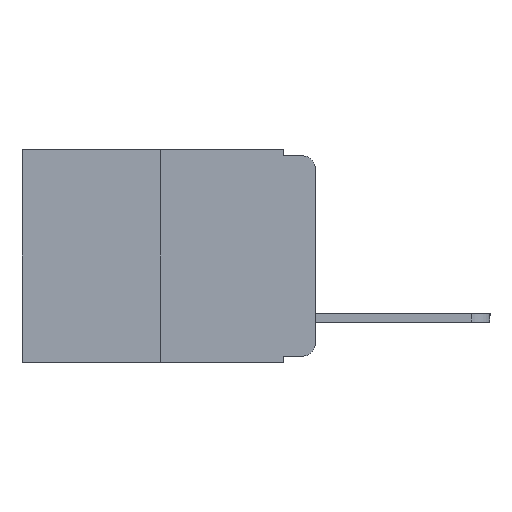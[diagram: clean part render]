
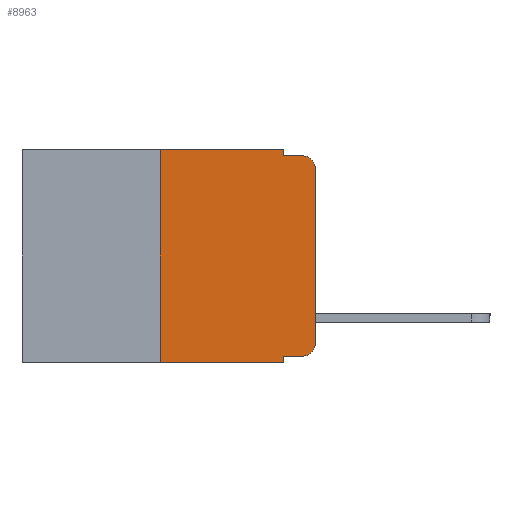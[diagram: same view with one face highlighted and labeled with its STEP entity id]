
A CAD part, left-side view. The second image highlights one B-rep face of the part: STEP entity #8963.
In plain terms, the highlighted planar face has unit normal (-1, 0, 0).
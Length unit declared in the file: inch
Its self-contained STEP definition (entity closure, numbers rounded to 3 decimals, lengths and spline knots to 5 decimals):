
#248 = CARTESIAN_POINT ( 'NONE',  ( 0., 0.02, -0.01 ) ) ;
#283 = VECTOR ( 'NONE', #9025, 39.37008 ) ;
#337 = CARTESIAN_POINT ( 'NONE',  ( 0., 0., -0.03 ) ) ;
#573 = LINE ( 'NONE', #3915, #283 ) ;
#720 = CARTESIAN_POINT ( 'NONE',  ( 0., 0.051, -0.01 ) ) ;
#937 = VECTOR ( 'NONE', #6327, 39.37008 ) ;
#947 = DIRECTION ( 'NONE',  ( 0., -1., 0. ) ) ;
#1385 = ORIENTED_EDGE ( 'NONE', *, *, #1768, .F. ) ;
#1392 = CARTESIAN_POINT ( 'NONE',  ( 0., 0.02, -0.03 ) ) ;
#1399 = VERTEX_POINT ( 'NONE', #7444 ) ;
#1763 = CARTESIAN_POINT ( 'NONE',  ( 0., 0., -0.313 ) ) ;
#1768 = EDGE_CURVE ( 'NONE', #5546, #5086, #3688, .T. ) ;
#1831 = CARTESIAN_POINT ( 'NONE',  ( 0., 0.051, -0.333 ) ) ;
#2217 = LINE ( 'NONE', #4560, #6785 ) ;
#2293 = VECTOR ( 'NONE', #9776, 39.37008 ) ;
#2401 = VERTEX_POINT ( 'NONE', #8206 ) ;
#2758 = EDGE_CURVE ( 'NONE', #6033, #5086, #10913, .T. ) ;
#2836 = CARTESIAN_POINT ( 'NONE',  ( 0., 0.25, 0. ) ) ;
#2842 = CARTESIAN_POINT ( 'NONE',  ( 0., 0.051, 0. ) ) ;
#2931 = VERTEX_POINT ( 'NONE', #1831 ) ;
#3153 = CARTESIAN_POINT ( 'NONE',  ( 0., 0.051, -0.343 ) ) ;
#3379 = EDGE_CURVE ( 'NONE', #5992, #6033, #8115, .T. ) ;
#3432 = PLANE ( 'NONE',  #9098 ) ;
#3538 = EDGE_CURVE ( 'NONE', #1399, #5992, #3868, .T. ) ;
#3688 = LINE ( 'NONE', #9476, #937 ) ;
#3834 = CARTESIAN_POINT ( 'NONE',  ( 0., 0.051, 0. ) ) ;
#3868 = CIRCLE ( 'NONE', #10484, 0.02 ) ;
#3899 = VERTEX_POINT ( 'NONE', #3153 ) ;
#3915 = CARTESIAN_POINT ( 'NONE',  ( 0., 0.051, -0.333 ) ) ;
#3979 = DIRECTION ( 'NONE',  ( 0., 0., -1. ) ) ;
#4302 = CARTESIAN_POINT ( 'NONE',  ( 0., 0.25, -0.343 ) ) ;
#4360 = EDGE_CURVE ( 'NONE', #2931, #1399, #573, .T. ) ;
#4463 = DIRECTION ( 'NONE',  ( 0., 0., 1. ) ) ;
#4489 = CARTESIAN_POINT ( 'NONE',  ( 0., 0., 0. ) ) ;
#4560 = CARTESIAN_POINT ( 'NONE',  ( 0., 0.25, 0. ) ) ;
#4561 = ORIENTED_EDGE ( 'NONE', *, *, #10525, .T. ) ;
#5086 = VERTEX_POINT ( 'NONE', #248 ) ;
#5288 = DIRECTION ( 'NONE',  ( 0., 0., -1. ) ) ;
#5478 = EDGE_CURVE ( 'NONE', #10217, #10529, #2217, .T. ) ;
#5546 = VERTEX_POINT ( 'NONE', #720 ) ;
#5595 = CARTESIAN_POINT ( 'NONE',  ( 0., 0.473, -0.343 ) ) ;
#5602 = EDGE_CURVE ( 'NONE', #2931, #3899, #10116, .T. ) ;
#5877 = VECTOR ( 'NONE', #947, 39.37008 ) ;
#5992 = VERTEX_POINT ( 'NONE', #1763 ) ;
#6033 = VERTEX_POINT ( 'NONE', #337 ) ;
#6080 = ORIENTED_EDGE ( 'NONE', *, *, #3379, .T. ) ;
#6327 = DIRECTION ( 'NONE',  ( 0., -1., 0. ) ) ;
#6343 = ORIENTED_EDGE ( 'NONE', *, *, #8007, .F. ) ;
#6396 = VECTOR ( 'NONE', #10530, 39.37008 ) ;
#6617 = ORIENTED_EDGE ( 'NONE', *, *, #10565, .F. ) ;
#6785 = VECTOR ( 'NONE', #10449, 39.37008 ) ;
#6878 = ORIENTED_EDGE ( 'NONE', *, *, #5602, .F. ) ;
#6937 = LINE ( 'NONE', #5595, #6396 ) ;
#6968 = CARTESIAN_POINT ( 'NONE',  ( 0., 0.473, 0. ) ) ;
#7144 = ORIENTED_EDGE ( 'NONE', *, *, #3538, .T. ) ;
#7434 = DIRECTION ( 'NONE',  ( -1., 0., 0. ) ) ;
#7444 = CARTESIAN_POINT ( 'NONE',  ( 0., 0.02, -0.333 ) ) ;
#7954 = VECTOR ( 'NONE', #9745, 39.37008 ) ;
#8007 = EDGE_CURVE ( 'NONE', #2401, #5546, #9046, .T. ) ;
#8082 = LINE ( 'NONE', #10593, #5877 ) ;
#8115 = LINE ( 'NONE', #4489, #8613 ) ;
#8206 = CARTESIAN_POINT ( 'NONE',  ( 0., 0.051, 0. ) ) ;
#8277 = ORIENTED_EDGE ( 'NONE', *, *, #2758, .T. ) ;
#8487 = FACE_OUTER_BOUND ( 'NONE', #9761, .T. ) ;
#8613 = VECTOR ( 'NONE', #4463, 39.37008 ) ;
#8963 = ADVANCED_FACE ( 'NONE', ( #8487 ), #3432, .F. ) ;
#9025 = DIRECTION ( 'NONE',  ( 0., -1., 0. ) ) ;
#9046 = LINE ( 'NONE', #3834, #2293 ) ;
#9098 = AXIS2_PLACEMENT_3D ( 'NONE', #6968, #10243, #5288 ) ;
#9476 = CARTESIAN_POINT ( 'NONE',  ( 0., 0.051, -0.01 ) ) ;
#9745 = DIRECTION ( 'NONE',  ( 0., 0., -1. ) ) ;
#9761 = EDGE_LOOP ( 'NONE', ( #6080, #8277, #1385, #6343, #6617, #10941, #4561, #6878, #11188, #7144 ) ) ;
#9776 = DIRECTION ( 'NONE',  ( 0., 0., -1. ) ) ;
#10116 = LINE ( 'NONE', #2842, #7954 ) ;
#10217 = VERTEX_POINT ( 'NONE', #4302 ) ;
#10243 = DIRECTION ( 'NONE',  ( 1., 0., 0. ) ) ;
#10404 = AXIS2_PLACEMENT_3D ( 'NONE', #1392, #7434, #3979 ) ;
#10449 = DIRECTION ( 'NONE',  ( 0., 0., 1. ) ) ;
#10484 = AXIS2_PLACEMENT_3D ( 'NONE', #10767, #10749, #10677 ) ;
#10525 = EDGE_CURVE ( 'NONE', #10217, #3899, #6937, .T. ) ;
#10529 = VERTEX_POINT ( 'NONE', #2836 ) ;
#10530 = DIRECTION ( 'NONE',  ( 0., -1., 0. ) ) ;
#10565 = EDGE_CURVE ( 'NONE', #10529, #2401, #8082, .T. ) ;
#10593 = CARTESIAN_POINT ( 'NONE',  ( 0., 0.473, 0. ) ) ;
#10677 = DIRECTION ( 'NONE',  ( 0., 0., -1. ) ) ;
#10749 = DIRECTION ( 'NONE',  ( -1., 0., 0. ) ) ;
#10767 = CARTESIAN_POINT ( 'NONE',  ( 0., 0.02, -0.313 ) ) ;
#10913 = CIRCLE ( 'NONE', #10404, 0.02 ) ;
#10941 = ORIENTED_EDGE ( 'NONE', *, *, #5478, .F. ) ;
#11188 = ORIENTED_EDGE ( 'NONE', *, *, #4360, .T. ) ;
